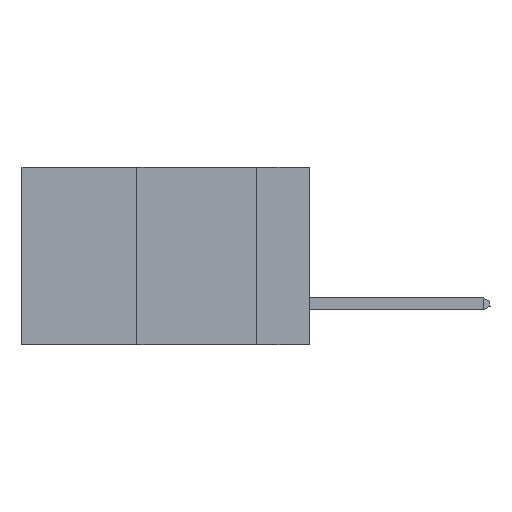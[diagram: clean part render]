
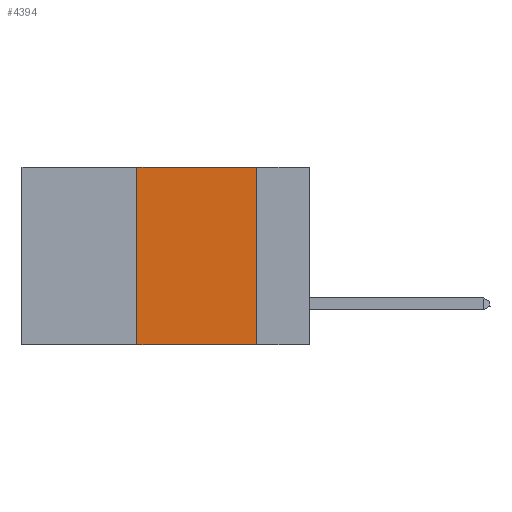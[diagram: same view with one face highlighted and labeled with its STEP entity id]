
A CAD part, left-side view. The second image highlights one B-rep face of the part: STEP entity #4394.
In plain terms, the highlighted planar face has unit normal (-1, 0, 0).
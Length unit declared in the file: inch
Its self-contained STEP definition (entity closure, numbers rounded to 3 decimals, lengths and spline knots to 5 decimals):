
#334 = AXIS2_PLACEMENT_3D ( 'NONE', #15084, #4417, #1044 ) ;
#492 = CARTESIAN_POINT ( 'NONE',  ( 0., 0.6, 0. ) ) ;
#531 = CARTESIAN_POINT ( 'NONE',  ( 0., 0.6, -0.37 ) ) ;
#622 = ORIENTED_EDGE ( 'NONE', *, *, #12654, .F. ) ;
#1044 = DIRECTION ( 'NONE',  ( 0., 0., -1. ) ) ;
#1656 = DIRECTION ( 'NONE',  ( 0., 0., -1. ) ) ;
#1997 = FACE_OUTER_BOUND ( 'NONE', #6325, .T. ) ;
#2650 = DIRECTION ( 'NONE',  ( 0., 0., 1. ) ) ;
#2678 = EDGE_CURVE ( 'NONE', #11749, #11063, #2829, .T. ) ;
#2725 = LINE ( 'NONE', #13332, #13691 ) ;
#2829 = LINE ( 'NONE', #492, #3797 ) ;
#2979 = ORIENTED_EDGE ( 'NONE', *, *, #6819, .T. ) ;
#3797 = VECTOR ( 'NONE', #6162, 39.37008 ) ;
#4394 = ADVANCED_FACE ( 'NONE', ( #1997 ), #5527, .F. ) ;
#4417 = DIRECTION ( 'NONE',  ( 1., 0., 0. ) ) ;
#4989 = ORIENTED_EDGE ( 'NONE', *, *, #2678, .F. ) ;
#5392 = LINE ( 'NONE', #531, #8343 ) ;
#5527 = PLANE ( 'NONE',  #334 ) ;
#6162 = DIRECTION ( 'NONE',  ( 0., -1., 0. ) ) ;
#6325 = EDGE_LOOP ( 'NONE', ( #6603, #4989, #622, #2979 ) ) ;
#6603 = ORIENTED_EDGE ( 'NONE', *, *, #9215, .F. ) ;
#6819 = EDGE_CURVE ( 'NONE', #8933, #7923, #5392, .T. ) ;
#7923 = VERTEX_POINT ( 'NONE', #14136 ) ;
#8069 = CARTESIAN_POINT ( 'NONE',  ( 0., 0.11, 0. ) ) ;
#8343 = VECTOR ( 'NONE', #8840, 39.37008 ) ;
#8810 = CARTESIAN_POINT ( 'NONE',  ( 0., 0.36, 0. ) ) ;
#8840 = DIRECTION ( 'NONE',  ( 0., -1., 0. ) ) ;
#8933 = VERTEX_POINT ( 'NONE', #13907 ) ;
#9215 = EDGE_CURVE ( 'NONE', #11063, #7923, #11077, .T. ) ;
#11063 = VERTEX_POINT ( 'NONE', #8069 ) ;
#11077 = LINE ( 'NONE', #12397, #13197 ) ;
#11749 = VERTEX_POINT ( 'NONE', #8810 ) ;
#12397 = CARTESIAN_POINT ( 'NONE',  ( 0., 0.11, 0. ) ) ;
#12654 = EDGE_CURVE ( 'NONE', #8933, #11749, #2725, .T. ) ;
#13197 = VECTOR ( 'NONE', #1656, 39.37008 ) ;
#13332 = CARTESIAN_POINT ( 'NONE',  ( 0., 0.36, 0. ) ) ;
#13691 = VECTOR ( 'NONE', #2650, 39.37008 ) ;
#13907 = CARTESIAN_POINT ( 'NONE',  ( 0., 0.36, -0.37 ) ) ;
#14136 = CARTESIAN_POINT ( 'NONE',  ( 0., 0.11, -0.37 ) ) ;
#15084 = CARTESIAN_POINT ( 'NONE',  ( 0., 0.6, 0. ) ) ;
